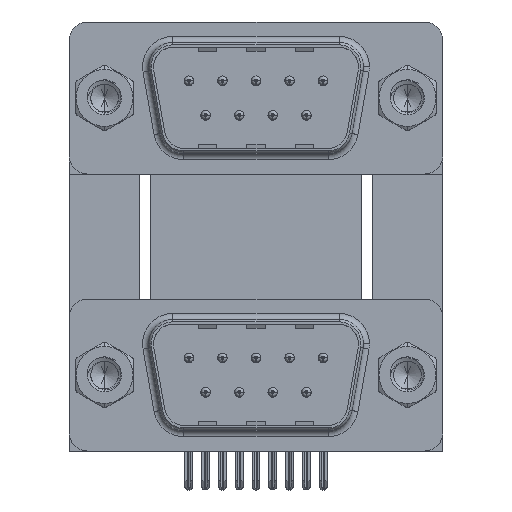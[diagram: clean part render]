
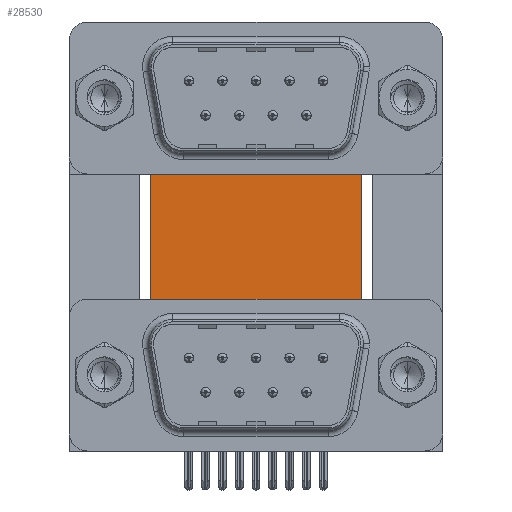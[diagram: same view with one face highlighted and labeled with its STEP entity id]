
A CAD part, top view. The second image highlights one B-rep face of the part: STEP entity #28530.
In plain terms, the highlighted planar face has unit normal (0, 0, 1).
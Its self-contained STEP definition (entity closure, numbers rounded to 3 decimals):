
#173 = VERTEX_POINT ( 'NONE', #25180 ) ;
#747 = CARTESIAN_POINT ( 'NONE',  ( 21.2, 16.585, -12. ) ) ;
#1441 = PLANE ( 'NONE',  #25660 ) ;
#3058 = CARTESIAN_POINT ( 'NONE',  ( 3.79, 16.585, -12. ) ) ;
#4390 = DIRECTION ( 'NONE',  ( -0.336, -0.942, 0. ) ) ;
#5642 = CARTESIAN_POINT ( 'NONE',  ( 2.9, -4.635, -12. ) ) ;
#6583 = EDGE_CURVE ( 'NONE', #6647, #29284, #8443, .T. ) ;
#6647 = VERTEX_POINT ( 'NONE', #29311 ) ;
#6944 = ORIENTED_EDGE ( 'NONE', *, *, #32187, .T. ) ;
#7633 = LINE ( 'NONE', #14680, #29723 ) ;
#7749 = VECTOR ( 'NONE', #24919, 1000. ) ;
#7798 = LINE ( 'NONE', #20003, #28704 ) ;
#7885 = LINE ( 'NONE', #23093, #26500 ) ;
#8406 = CARTESIAN_POINT ( 'NONE',  ( 22.09, -4.635, -12. ) ) ;
#8443 = LINE ( 'NONE', #747, #25441 ) ;
#8839 = VECTOR ( 'NONE', #14591, 1000. ) ;
#9332 = VECTOR ( 'NONE', #23763, 1000. ) ;
#9554 = LINE ( 'NONE', #19746, #7749 ) ;
#9996 = EDGE_CURVE ( 'NONE', #173, #6647, #21433, .T. ) ;
#10381 = CARTESIAN_POINT ( 'NONE',  ( 22.09, -3.735, -12. ) ) ;
#11634 = FACE_OUTER_BOUND ( 'NONE', #24051, .T. ) ;
#11701 = CARTESIAN_POINT ( 'NONE',  ( 2.4, -4.635, -12. ) ) ;
#12532 = EDGE_CURVE ( 'NONE', #28204, #27116, #32291, .T. ) ;
#12808 = EDGE_CURVE ( 'NONE', #14024, #29098, #19386, .T. ) ;
#13731 = VECTOR ( 'NONE', #4390, 1000. ) ;
#14024 = VERTEX_POINT ( 'NONE', #10381 ) ;
#14269 = LINE ( 'NONE', #27321, #8839 ) ;
#14430 = VERTEX_POINT ( 'NONE', #32319 ) ;
#14591 = DIRECTION ( 'NONE',  ( 1., 0., 0. ) ) ;
#14680 = CARTESIAN_POINT ( 'NONE',  ( 2.9, -4.635, -12. ) ) ;
#14686 = ORIENTED_EDGE ( 'NONE', *, *, #31024, .T. ) ;
#15009 = CARTESIAN_POINT ( 'NONE',  ( 3.79, -0.735, -12. ) ) ;
#15480 = DIRECTION ( 'NONE',  ( 0., -1., 0. ) ) ;
#15751 = ORIENTED_EDGE ( 'NONE', *, *, #12808, .T. ) ;
#15849 = VECTOR ( 'NONE', #22055, 1000. ) ;
#16396 = EDGE_CURVE ( 'NONE', #27116, #18257, #7633, .T. ) ;
#16482 = DIRECTION ( 'NONE',  ( -1., 0., 0. ) ) ;
#16637 = ORIENTED_EDGE ( 'NONE', *, *, #30086, .T. ) ;
#16898 = CARTESIAN_POINT ( 'NONE',  ( 21.2, -0.735, -12. ) ) ;
#16918 = CARTESIAN_POINT ( 'NONE',  ( 2.4, -4.635, -12. ) ) ;
#16988 = DIRECTION ( 'NONE',  ( 0., 0., -1. ) ) ;
#17860 = VECTOR ( 'NONE', #22997, 1000. ) ;
#18257 = VERTEX_POINT ( 'NONE', #5642 ) ;
#18863 = ORIENTED_EDGE ( 'NONE', *, *, #6583, .F. ) ;
#19386 = LINE ( 'NONE', #24572, #15849 ) ;
#19746 = CARTESIAN_POINT ( 'NONE',  ( 2.9, -3.735, -12. ) ) ;
#19979 = LINE ( 'NONE', #20158, #17860 ) ;
#20003 = CARTESIAN_POINT ( 'NONE',  ( 3.79, 16.585, -12. ) ) ;
#20158 = CARTESIAN_POINT ( 'NONE',  ( 22.59, -4.635, -12. ) ) ;
#20926 = DIRECTION ( 'NONE',  ( 1., 0., 0. ) ) ;
#21433 = LINE ( 'NONE', #3058, #9332 ) ;
#22055 = DIRECTION ( 'NONE',  ( 0., -1., 0. ) ) ;
#22915 = EDGE_CURVE ( 'NONE', #173, #28204, #7798, .T. ) ;
#22997 = DIRECTION ( 'NONE',  ( -0.336, 0.942, 0. ) ) ;
#23093 = CARTESIAN_POINT ( 'NONE',  ( 22.09, -4.635, -12. ) ) ;
#23763 = DIRECTION ( 'NONE',  ( 1., 0., 0. ) ) ;
#23966 = DIRECTION ( 'NONE',  ( 0., -1., 0. ) ) ;
#24051 = EDGE_LOOP ( 'NONE', ( #14686, #15751, #6944, #28138, #18863, #27078, #33001, #32136, #32157, #16637 ) ) ;
#24333 = CARTESIAN_POINT ( 'NONE',  ( 3.79, 16.585, -12. ) ) ;
#24572 = CARTESIAN_POINT ( 'NONE',  ( 22.09, -3.735, -12. ) ) ;
#24919 = DIRECTION ( 'NONE',  ( 0., 1., 0. ) ) ;
#25180 = CARTESIAN_POINT ( 'NONE',  ( 3.79, 16.585, -12. ) ) ;
#25441 = VECTOR ( 'NONE', #23966, 1000. ) ;
#25660 = AXIS2_PLACEMENT_3D ( 'NONE', #24333, #16988, #16482 ) ;
#26500 = VECTOR ( 'NONE', #20926, 1000. ) ;
#26540 = VERTEX_POINT ( 'NONE', #30866 ) ;
#27078 = ORIENTED_EDGE ( 'NONE', *, *, #9996, .F. ) ;
#27116 = VERTEX_POINT ( 'NONE', #11701 ) ;
#27321 = CARTESIAN_POINT ( 'NONE',  ( 3.79, -3.735, -12. ) ) ;
#28138 = ORIENTED_EDGE ( 'NONE', *, *, #29804, .T. ) ;
#28204 = VERTEX_POINT ( 'NONE', #15009 ) ;
#28530 = ADVANCED_FACE ( 'NONE', ( #11634 ), #1441, .F. ) ;
#28704 = VECTOR ( 'NONE', #15480, 1000. ) ;
#29098 = VERTEX_POINT ( 'NONE', #8406 ) ;
#29284 = VERTEX_POINT ( 'NONE', #16898 ) ;
#29311 = CARTESIAN_POINT ( 'NONE',  ( 21.2, 16.585, -12. ) ) ;
#29723 = VECTOR ( 'NONE', #29744, 1000. ) ;
#29744 = DIRECTION ( 'NONE',  ( 1., 0., 0. ) ) ;
#29804 = EDGE_CURVE ( 'NONE', #14430, #29284, #19979, .T. ) ;
#30086 = EDGE_CURVE ( 'NONE', #18257, #26540, #9554, .T. ) ;
#30866 = CARTESIAN_POINT ( 'NONE',  ( 2.9, -3.735, -12. ) ) ;
#31024 = EDGE_CURVE ( 'NONE', #26540, #14024, #14269, .T. ) ;
#32136 = ORIENTED_EDGE ( 'NONE', *, *, #12532, .T. ) ;
#32157 = ORIENTED_EDGE ( 'NONE', *, *, #16396, .T. ) ;
#32187 = EDGE_CURVE ( 'NONE', #29098, #14430, #7885, .T. ) ;
#32291 = LINE ( 'NONE', #16918, #13731 ) ;
#32319 = CARTESIAN_POINT ( 'NONE',  ( 22.59, -4.635, -12. ) ) ;
#33001 = ORIENTED_EDGE ( 'NONE', *, *, #22915, .T. ) ;
